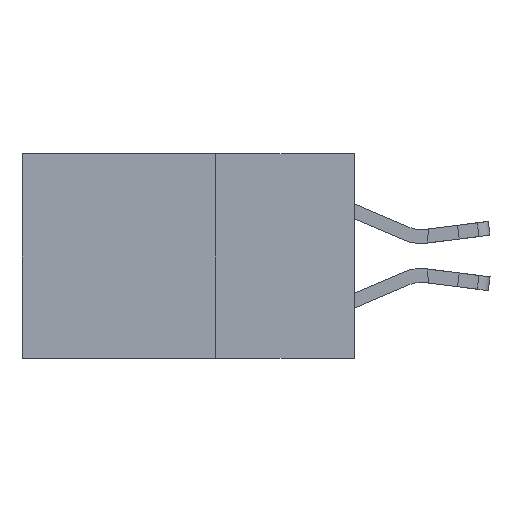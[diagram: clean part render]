
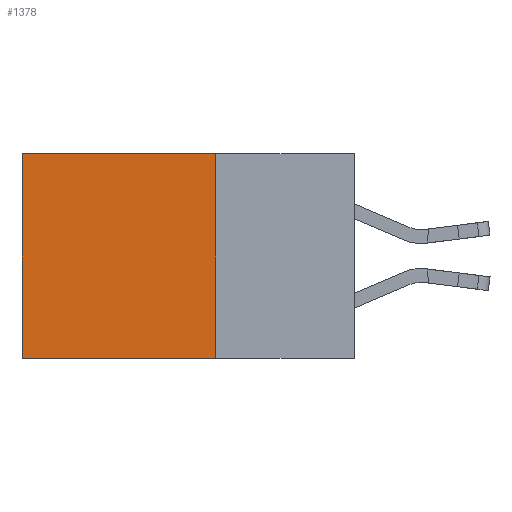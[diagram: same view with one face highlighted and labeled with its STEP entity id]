
A CAD part, left-side view. The second image highlights one B-rep face of the part: STEP entity #1378.
In plain terms, the highlighted planar face has unit normal (-1, 0, 0).
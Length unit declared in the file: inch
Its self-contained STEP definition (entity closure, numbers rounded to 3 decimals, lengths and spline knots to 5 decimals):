
#62 = LINE ( 'NONE', #20593, #7061 ) ;
#102 = VECTOR ( 'NONE', #3719, 39.37008 ) ;
#1378 = ADVANCED_FACE ( 'NONE', ( #12630 ), #19009, .F. ) ;
#1526 = VERTEX_POINT ( 'NONE', #11035 ) ;
#1759 = EDGE_LOOP ( 'NONE', ( #4636, #16479, #11680, #21634 ) ) ;
#3072 = DIRECTION ( 'NONE',  ( 1., 0., 0. ) ) ;
#3719 = DIRECTION ( 'NONE',  ( 0., 1., 0. ) ) ;
#4267 = DIRECTION ( 'NONE',  ( 0., 1., 0. ) ) ;
#4636 = ORIENTED_EDGE ( 'NONE', *, *, #11682, .T. ) ;
#4882 = CARTESIAN_POINT ( 'NONE',  ( 0.2615, 0.25, -0.37 ) ) ;
#5630 = CARTESIAN_POINT ( 'NONE',  ( 0.2615, 0.6, -0.37 ) ) ;
#7026 = VERTEX_POINT ( 'NONE', #15778 ) ;
#7061 = VECTOR ( 'NONE', #12064, 39.37008 ) ;
#7235 = EDGE_CURVE ( 'NONE', #12316, #7897, #13989, .T. ) ;
#7897 = VERTEX_POINT ( 'NONE', #21782 ) ;
#9159 = LINE ( 'NONE', #5630, #17694 ) ;
#9282 = AXIS2_PLACEMENT_3D ( 'NONE', #4882, #3072, #16143 ) ;
#11035 = CARTESIAN_POINT ( 'NONE',  ( 0.2615, 0.6, -0.37 ) ) ;
#11585 = EDGE_CURVE ( 'NONE', #7026, #1526, #21856, .T. ) ;
#11680 = ORIENTED_EDGE ( 'NONE', *, *, #16641, .F. ) ;
#11682 = EDGE_CURVE ( 'NONE', #7897, #1526, #9159, .T. ) ;
#12064 = DIRECTION ( 'NONE',  ( 0., 0., -1. ) ) ;
#12316 = VERTEX_POINT ( 'NONE', #12590 ) ;
#12590 = CARTESIAN_POINT ( 'NONE',  ( 0.2615, 0.25, 0. ) ) ;
#12630 = FACE_OUTER_BOUND ( 'NONE', #1759, .T. ) ;
#13989 = LINE ( 'NONE', #16246, #18570 ) ;
#15660 = CARTESIAN_POINT ( 'NONE',  ( 0.2615, 0.25, -0.37 ) ) ;
#15778 = CARTESIAN_POINT ( 'NONE',  ( 0.2615, 0.25, -0.37 ) ) ;
#16143 = DIRECTION ( 'NONE',  ( 0., 0., -1. ) ) ;
#16246 = CARTESIAN_POINT ( 'NONE',  ( 0.2615, 0.25, 0. ) ) ;
#16479 = ORIENTED_EDGE ( 'NONE', *, *, #11585, .F. ) ;
#16641 = EDGE_CURVE ( 'NONE', #12316, #7026, #62, .T. ) ;
#17694 = VECTOR ( 'NONE', #19331, 39.37008 ) ;
#18570 = VECTOR ( 'NONE', #4267, 39.37008 ) ;
#19009 = PLANE ( 'NONE',  #9282 ) ;
#19331 = DIRECTION ( 'NONE',  ( 0., 0., -1. ) ) ;
#20593 = CARTESIAN_POINT ( 'NONE',  ( 0.2615, 0.25, -0.37 ) ) ;
#21634 = ORIENTED_EDGE ( 'NONE', *, *, #7235, .T. ) ;
#21782 = CARTESIAN_POINT ( 'NONE',  ( 0.2615, 0.6, 0. ) ) ;
#21856 = LINE ( 'NONE', #15660, #102 ) ;
